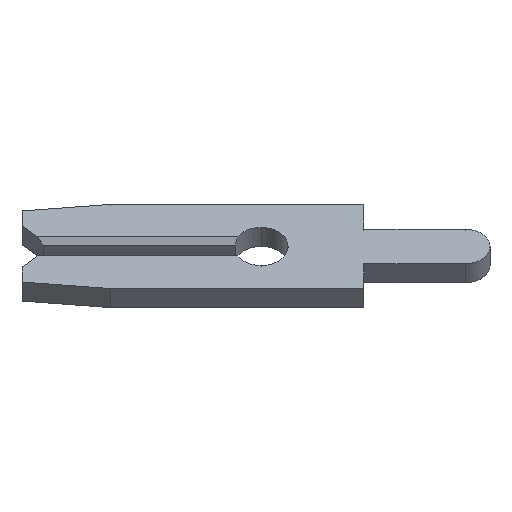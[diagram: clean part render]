
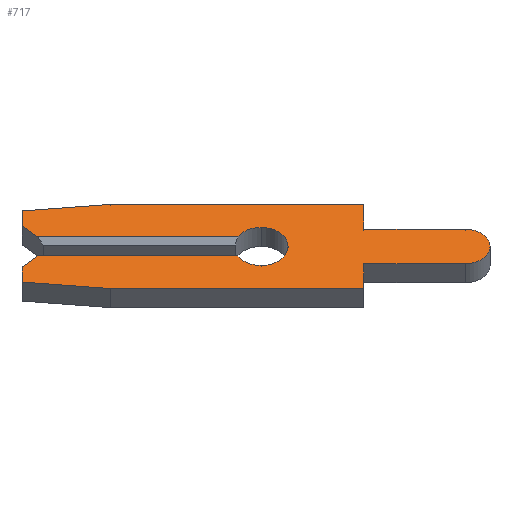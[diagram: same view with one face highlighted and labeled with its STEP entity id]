
A CAD part, left-side view. The second image highlights one B-rep face of the part: STEP entity #717.
In plain terms, the highlighted face is planar.
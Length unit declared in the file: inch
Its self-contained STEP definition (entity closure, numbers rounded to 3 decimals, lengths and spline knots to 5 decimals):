
#4 = FACE_OUTER_BOUND ( 'NONE', #181, .T. ) ;
#5 = AXIS2_PLACEMENT_3D ( 'NONE', #492, #726, #69 ) ;
#6 = DIRECTION ( 'NONE',  ( 0., -0.707, 0.707 ) ) ;
#12 = VECTOR ( 'NONE', #536, 39.37008 ) ;
#33 = EDGE_CURVE ( 'NONE', #316, #283, #964, .T. ) ;
#50 = ORIENTED_EDGE ( 'NONE', *, *, #849, .F. ) ;
#55 = DIRECTION ( 'NONE',  ( 0., -0.995, 0.105 ) ) ;
#64 = CARTESIAN_POINT ( 'NONE',  ( -0.013, 0.231, 0.04857 ) ) ;
#69 = DIRECTION ( 'NONE',  ( 0., 0., -1. ) ) ;
#71 = DIRECTION ( 'NONE',  ( 0., 0., -1. ) ) ;
#72 = CARTESIAN_POINT ( 'NONE',  ( -0.013, 0., 0.026 ) ) ;
#76 = VECTOR ( 'NONE', #892, 39.37008 ) ;
#84 = CARTESIAN_POINT ( 'NONE',  ( -0.013, 0.231, -0.04857 ) ) ;
#92 = ORIENTED_EDGE ( 'NONE', *, *, #33, .F. ) ;
#94 = CARTESIAN_POINT ( 'NONE',  ( -0.013, -0.099, -0.0575 ) ) ;
#102 = CARTESIAN_POINT ( 'NONE',  ( -0.013, 0., 0. ) ) ;
#110 = CARTESIAN_POINT ( 'NONE',  ( -0.013, -0.099, 0.0235 ) ) ;
#120 = EDGE_CURVE ( 'NONE', #816, #830, #574, .T. ) ;
#136 = VECTOR ( 'NONE', #287, 39.37008 ) ;
#140 = CIRCLE ( 'NONE', #388, 0.0235 ) ;
#142 = DIRECTION ( 'NONE',  ( -1., 0., 0. ) ) ;
#144 = EDGE_CURVE ( 'NONE', #512, #316, #350, .T. ) ;
#146 = CARTESIAN_POINT ( 'NONE',  ( -0.013, 0., 0. ) ) ;
#151 = VECTOR ( 'NONE', #834, 39.37008 ) ;
#157 = CARTESIAN_POINT ( 'NONE',  ( -0.013, 0.146, 0.0575 ) ) ;
#170 = CARTESIAN_POINT ( 'NONE',  ( -0.013, 0., -0.026 ) ) ;
#181 = EDGE_LOOP ( 'NONE', ( #417, #501, #211, #50, #755, #432, #92, #919, #404, #396, #460, #418, #1049, #395, #844, #882, #284, #915 ) ) ;
#196 = VERTEX_POINT ( 'NONE', #826 ) ;
#205 = CARTESIAN_POINT ( 'NONE',  ( -0.013, 0.02252, -0.013 ) ) ;
#210 = VERTEX_POINT ( 'NONE', #72 ) ;
#211 = ORIENTED_EDGE ( 'NONE', *, *, #831, .F. ) ;
#225 = AXIS2_PLACEMENT_3D ( 'NONE', #572, #142, #721 ) ;
#228 = CARTESIAN_POINT ( 'NONE',  ( -0.013, -0.1975, -0.0235 ) ) ;
#233 = EDGE_CURVE ( 'NONE', #245, #727, #787, .T. ) ;
#245 = VERTEX_POINT ( 'NONE', #409 ) ;
#250 = CARTESIAN_POINT ( 'NONE',  ( -0.013, 0.216, 0.013 ) ) ;
#264 = DIRECTION ( 'NONE',  ( 1., 0., 0. ) ) ;
#272 = EDGE_CURVE ( 'NONE', #472, #816, #140, .T. ) ;
#283 = VERTEX_POINT ( 'NONE', #426 ) ;
#284 = ORIENTED_EDGE ( 'NONE', *, *, #369, .F. ) ;
#287 = DIRECTION ( 'NONE',  ( 0., 0., -1. ) ) ;
#289 = EDGE_CURVE ( 'NONE', #283, #489, #470, .T. ) ;
#294 = LINE ( 'NONE', #946, #566 ) ;
#301 = VERTEX_POINT ( 'NONE', #94 ) ;
#303 = EDGE_CURVE ( 'NONE', #489, #513, #361, .T. ) ;
#308 = EDGE_CURVE ( 'NONE', #210, #766, #1036, .T. ) ;
#314 = DIRECTION ( 'NONE',  ( 0., -1., 0. ) ) ;
#316 = VERTEX_POINT ( 'NONE', #435 ) ;
#329 = CIRCLE ( 'NONE', #743, 0.026 ) ;
#349 = CARTESIAN_POINT ( 'NONE',  ( -0.013, 0.2105, -0.0075 ) ) ;
#350 = LINE ( 'NONE', #84, #151 ) ;
#361 = LINE ( 'NONE', #1002, #993 ) ;
#369 = EDGE_CURVE ( 'NONE', #196, #473, #655, .T. ) ;
#388 = AXIS2_PLACEMENT_3D ( 'NONE', #520, #264, #590 ) ;
#395 = ORIENTED_EDGE ( 'NONE', *, *, #475, .F. ) ;
#396 = ORIENTED_EDGE ( 'NONE', *, *, #542, .F. ) ;
#404 = ORIENTED_EDGE ( 'NONE', *, *, #555, .F. ) ;
#409 = CARTESIAN_POINT ( 'NONE',  ( -0.013, 0.146, 0.0575 ) ) ;
#417 = ORIENTED_EDGE ( 'NONE', *, *, #866, .T. ) ;
#418 = ORIENTED_EDGE ( 'NONE', *, *, #272, .F. ) ;
#426 = CARTESIAN_POINT ( 'NONE',  ( -0.013, 0.231, -0.028 ) ) ;
#432 = ORIENTED_EDGE ( 'NONE', *, *, #289, .F. ) ;
#435 = CARTESIAN_POINT ( 'NONE',  ( -0.013, 0.231, -0.04857 ) ) ;
#439 = DIRECTION ( 'NONE',  ( 0., -1., 0. ) ) ;
#460 = ORIENTED_EDGE ( 'NONE', *, *, #120, .F. ) ;
#470 = LINE ( 'NONE', #349, #559 ) ;
#472 = VERTEX_POINT ( 'NONE', #1012 ) ;
#473 = VERTEX_POINT ( 'NONE', #689 ) ;
#475 = EDGE_CURVE ( 'NONE', #727, #776, #812, .T. ) ;
#482 = EDGE_CURVE ( 'NONE', #776, #472, #682, .T. ) ;
#483 = CARTESIAN_POINT ( 'NONE',  ( -0.013, -0.099, -0.0235 ) ) ;
#487 = CARTESIAN_POINT ( 'NONE',  ( -0.013, -0.099, 0.0575 ) ) ;
#489 = VERTEX_POINT ( 'NONE', #533 ) ;
#492 = CARTESIAN_POINT ( 'NONE',  ( -0.013, 0., 0. ) ) ;
#495 = DIRECTION ( 'NONE',  ( 0., 1., 0. ) ) ;
#501 = ORIENTED_EDGE ( 'NONE', *, *, #308, .F. ) ;
#505 = EDGE_CURVE ( 'NONE', #880, #196, #294, .T. ) ;
#512 = VERTEX_POINT ( 'NONE', #771 ) ;
#513 = VERTEX_POINT ( 'NONE', #205 ) ;
#517 = DIRECTION ( 'NONE',  ( 0., 0., -1. ) ) ;
#520 = CARTESIAN_POINT ( 'NONE',  ( -0.013, -0.1975, 0. ) ) ;
#533 = CARTESIAN_POINT ( 'NONE',  ( -0.013, 0.216, -0.013 ) ) ;
#536 = DIRECTION ( 'NONE',  ( 0., 1., 0. ) ) ;
#542 = EDGE_CURVE ( 'NONE', #830, #301, #824, .T. ) ;
#553 = VECTOR ( 'NONE', #314, 39.37008 ) ;
#555 = EDGE_CURVE ( 'NONE', #301, #512, #926, .T. ) ;
#559 = VECTOR ( 'NONE', #6, 39.37008 ) ;
#562 = CARTESIAN_POINT ( 'NONE',  ( -0.013, 0.231, 0.013 ) ) ;
#566 = VECTOR ( 'NONE', #701, 39.37008 ) ;
#572 = CARTESIAN_POINT ( 'NONE',  ( -0.013, 0., 0. ) ) ;
#573 = VECTOR ( 'NONE', #745, 39.37008 ) ;
#574 = LINE ( 'NONE', #483, #750 ) ;
#590 = DIRECTION ( 'NONE',  ( 0., 0., 1. ) ) ;
#594 = DIRECTION ( 'NONE',  ( 0., 0., 1. ) ) ;
#606 = CARTESIAN_POINT ( 'NONE',  ( -0.013, 0.146, -0.0575 ) ) ;
#639 = LINE ( 'NONE', #64, #1053 ) ;
#640 = CARTESIAN_POINT ( 'NONE',  ( -0.013, 0.02252, 0.013 ) ) ;
#655 = LINE ( 'NONE', #846, #899 ) ;
#682 = LINE ( 'NONE', #110, #782 ) ;
#689 = CARTESIAN_POINT ( 'NONE',  ( -0.013, 0.231, 0.04857 ) ) ;
#701 = DIRECTION ( 'NONE',  ( 0., 0.707, 0.707 ) ) ;
#717 = ADVANCED_FACE ( 'NONE', ( #4 ), #1060, .F. ) ;
#720 = CARTESIAN_POINT ( 'NONE',  ( -0.013, 0.231, -0.028 ) ) ;
#721 = DIRECTION ( 'NONE',  ( 0., 0., -1. ) ) ;
#726 = DIRECTION ( 'NONE',  ( 1., 0., 0. ) ) ;
#727 = VERTEX_POINT ( 'NONE', #487 ) ;
#732 = DIRECTION ( 'NONE',  ( -1., 0., 0. ) ) ;
#743 = AXIS2_PLACEMENT_3D ( 'NONE', #146, #732, #71 ) ;
#745 = DIRECTION ( 'NONE',  ( 0., -1., 0. ) ) ;
#750 = VECTOR ( 'NONE', #495, 39.37008 ) ;
#755 = ORIENTED_EDGE ( 'NONE', *, *, #303, .F. ) ;
#766 = VERTEX_POINT ( 'NONE', #640 ) ;
#767 = CIRCLE ( 'NONE', #225, 0.026 ) ;
#771 = CARTESIAN_POINT ( 'NONE',  ( -0.013, 0.146, -0.0575 ) ) ;
#776 = VERTEX_POINT ( 'NONE', #811 ) ;
#778 = LINE ( 'NONE', #562, #553 ) ;
#782 = VECTOR ( 'NONE', #851, 39.37008 ) ;
#787 = LINE ( 'NONE', #157, #573 ) ;
#794 = EDGE_CURVE ( 'NONE', #473, #245, #639, .T. ) ;
#811 = CARTESIAN_POINT ( 'NONE',  ( -0.013, -0.099, 0.0235 ) ) ;
#812 = LINE ( 'NONE', #942, #897 ) ;
#816 = VERTEX_POINT ( 'NONE', #228 ) ;
#817 = CARTESIAN_POINT ( 'NONE',  ( -0.013, -0.099, -0.0235 ) ) ;
#824 = LINE ( 'NONE', #1020, #136 ) ;
#826 = CARTESIAN_POINT ( 'NONE',  ( -0.013, 0.231, 0.028 ) ) ;
#830 = VERTEX_POINT ( 'NONE', #817 ) ;
#831 = EDGE_CURVE ( 'NONE', #905, #210, #329, .T. ) ;
#834 = DIRECTION ( 'NONE',  ( 0., 0.995, 0.105 ) ) ;
#844 = ORIENTED_EDGE ( 'NONE', *, *, #233, .F. ) ;
#846 = CARTESIAN_POINT ( 'NONE',  ( -0.013, 0.231, 0.028 ) ) ;
#848 = DIRECTION ( 'NONE',  ( -1., 0., 0. ) ) ;
#849 = EDGE_CURVE ( 'NONE', #513, #905, #767, .T. ) ;
#851 = DIRECTION ( 'NONE',  ( 0., -1., 0. ) ) ;
#859 = DIRECTION ( 'NONE',  ( 0., 0., -1. ) ) ;
#866 = EDGE_CURVE ( 'NONE', #880, #766, #778, .T. ) ;
#880 = VERTEX_POINT ( 'NONE', #250 ) ;
#882 = ORIENTED_EDGE ( 'NONE', *, *, #794, .F. ) ;
#892 = DIRECTION ( 'NONE',  ( 0., 0., 1. ) ) ;
#897 = VECTOR ( 'NONE', #859, 39.37008 ) ;
#899 = VECTOR ( 'NONE', #594, 39.37008 ) ;
#905 = VERTEX_POINT ( 'NONE', #170 ) ;
#915 = ORIENTED_EDGE ( 'NONE', *, *, #505, .F. ) ;
#919 = ORIENTED_EDGE ( 'NONE', *, *, #144, .F. ) ;
#926 = LINE ( 'NONE', #606, #12 ) ;
#942 = CARTESIAN_POINT ( 'NONE',  ( -0.013, -0.099, 0.0575 ) ) ;
#946 = CARTESIAN_POINT ( 'NONE',  ( -0.013, 0.2105, 0.0075 ) ) ;
#954 = AXIS2_PLACEMENT_3D ( 'NONE', #102, #848, #517 ) ;
#964 = LINE ( 'NONE', #720, #76 ) ;
#993 = VECTOR ( 'NONE', #439, 39.37008 ) ;
#1002 = CARTESIAN_POINT ( 'NONE',  ( -0.013, 0., -0.013 ) ) ;
#1012 = CARTESIAN_POINT ( 'NONE',  ( -0.013, -0.1975, 0.0235 ) ) ;
#1020 = CARTESIAN_POINT ( 'NONE',  ( -0.013, -0.099, -0.0575 ) ) ;
#1036 = CIRCLE ( 'NONE', #954, 0.026 ) ;
#1049 = ORIENTED_EDGE ( 'NONE', *, *, #482, .F. ) ;
#1053 = VECTOR ( 'NONE', #55, 39.37008 ) ;
#1060 = PLANE ( 'NONE',  #5 ) ;
